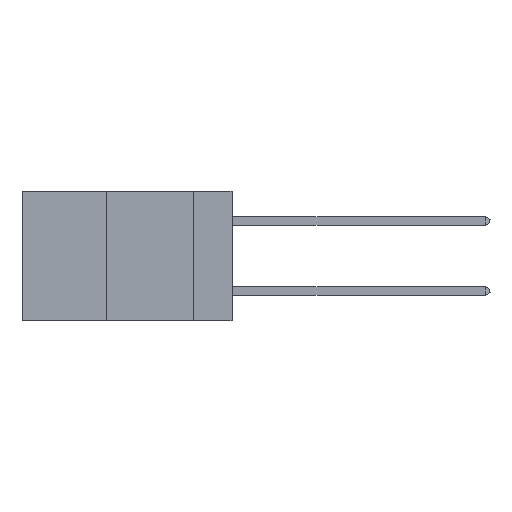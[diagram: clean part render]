
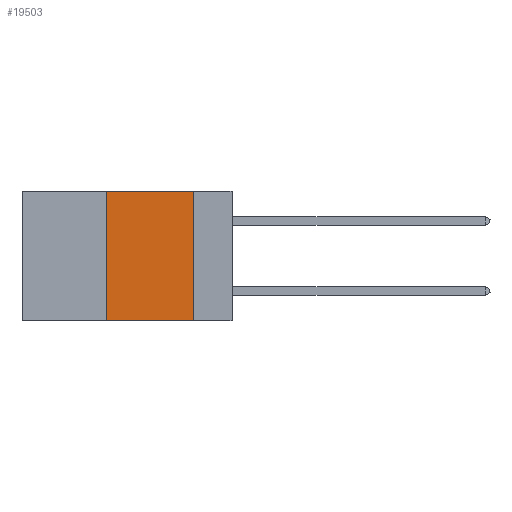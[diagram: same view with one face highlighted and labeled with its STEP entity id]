
A CAD part, left-side view. The second image highlights one B-rep face of the part: STEP entity #19503.
In plain terms, the highlighted planar face has unit normal (-1, 0, 0).
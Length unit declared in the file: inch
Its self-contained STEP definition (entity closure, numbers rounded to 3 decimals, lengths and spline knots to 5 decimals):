
#464 = CARTESIAN_POINT ( 'NONE',  ( 0., 0.11, 0. ) ) ;
#1889 = LINE ( 'NONE', #18423, #16900 ) ;
#4109 = DIRECTION ( 'NONE',  ( 1., 0., 0. ) ) ;
#5053 = ORIENTED_EDGE ( 'NONE', *, *, #13615, .F. ) ;
#5162 = CARTESIAN_POINT ( 'NONE',  ( 0., 0.11, -0.37 ) ) ;
#6004 = CARTESIAN_POINT ( 'NONE',  ( 0., 0.11, 0. ) ) ;
#6819 = CARTESIAN_POINT ( 'NONE',  ( 0., 0.6, -0.37 ) ) ;
#6873 = VECTOR ( 'NONE', #8777, 39.37008 ) ;
#8777 = DIRECTION ( 'NONE',  ( 0., -1., 0. ) ) ;
#9541 = EDGE_CURVE ( 'NONE', #13496, #11291, #1889, .T. ) ;
#10018 = AXIS2_PLACEMENT_3D ( 'NONE', #21533, #4109, #17756 ) ;
#10524 = DIRECTION ( 'NONE',  ( 0., 0., -1. ) ) ;
#10803 = FACE_OUTER_BOUND ( 'NONE', #15531, .T. ) ;
#11291 = VERTEX_POINT ( 'NONE', #12948 ) ;
#11899 = CARTESIAN_POINT ( 'NONE',  ( 0., 0.6, 0. ) ) ;
#12172 = EDGE_CURVE ( 'NONE', #11291, #18869, #21761, .T. ) ;
#12948 = CARTESIAN_POINT ( 'NONE',  ( 0., 0.36, 0. ) ) ;
#13496 = VERTEX_POINT ( 'NONE', #14116 ) ;
#13615 = EDGE_CURVE ( 'NONE', #18869, #18048, #15359, .T. ) ;
#13852 = DIRECTION ( 'NONE',  ( 0., -1., 0. ) ) ;
#13998 = ORIENTED_EDGE ( 'NONE', *, *, #9541, .F. ) ;
#14116 = CARTESIAN_POINT ( 'NONE',  ( 0., 0.36, -0.37 ) ) ;
#14750 = DIRECTION ( 'NONE',  ( 0., 0., 1. ) ) ;
#15359 = LINE ( 'NONE', #464, #25028 ) ;
#15531 = EDGE_LOOP ( 'NONE', ( #5053, #17206, #13998, #19918 ) ) ;
#16900 = VECTOR ( 'NONE', #14750, 39.37008 ) ;
#17206 = ORIENTED_EDGE ( 'NONE', *, *, #12172, .F. ) ;
#17239 = LINE ( 'NONE', #6819, #6873 ) ;
#17256 = VECTOR ( 'NONE', #13852, 39.37008 ) ;
#17756 = DIRECTION ( 'NONE',  ( 0., 0., -1. ) ) ;
#17945 = EDGE_CURVE ( 'NONE', #13496, #18048, #17239, .T. ) ;
#18048 = VERTEX_POINT ( 'NONE', #5162 ) ;
#18423 = CARTESIAN_POINT ( 'NONE',  ( 0., 0.36, 0. ) ) ;
#18869 = VERTEX_POINT ( 'NONE', #6004 ) ;
#19503 = ADVANCED_FACE ( 'NONE', ( #10803 ), #23490, .F. ) ;
#19918 = ORIENTED_EDGE ( 'NONE', *, *, #17945, .T. ) ;
#21533 = CARTESIAN_POINT ( 'NONE',  ( 0., 0.6, 0. ) ) ;
#21761 = LINE ( 'NONE', #11899, #17256 ) ;
#23490 = PLANE ( 'NONE',  #10018 ) ;
#25028 = VECTOR ( 'NONE', #10524, 39.37008 ) ;
